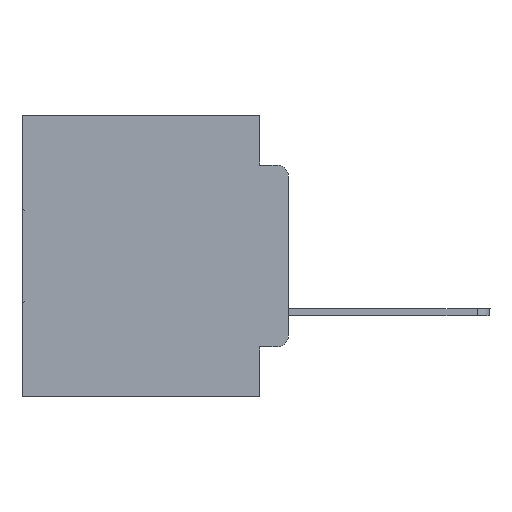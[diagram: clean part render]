
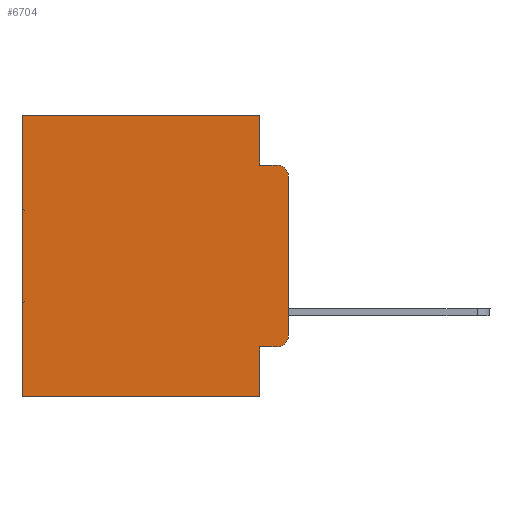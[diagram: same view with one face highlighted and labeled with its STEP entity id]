
A CAD part, left-side view. The second image highlights one B-rep face of the part: STEP entity #6704.
In plain terms, the highlighted planar face has unit normal (-1, 0, 0).
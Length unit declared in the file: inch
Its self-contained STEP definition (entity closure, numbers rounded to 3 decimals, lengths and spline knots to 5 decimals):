
#90 = AXIS2_PLACEMENT_3D ( 'NONE', #8830, #5706, #25961 ) ;
#226 = DIRECTION ( 'NONE',  ( 0., 0., -1. ) ) ;
#318 = DIRECTION ( 'NONE',  ( 0., -1., 0. ) ) ;
#377 = ORIENTED_EDGE ( 'NONE', *, *, #26750, .F. ) ;
#945 = EDGE_CURVE ( 'NONE', #11277, #2841, #8264, .T. ) ;
#1749 = VECTOR ( 'NONE', #15007, 39.37008 ) ;
#2358 = VERTEX_POINT ( 'NONE', #23683 ) ;
#2548 = DIRECTION ( 'NONE',  ( -1., 0., 0. ) ) ;
#2841 = VERTEX_POINT ( 'NONE', #30190 ) ;
#4095 = VERTEX_POINT ( 'NONE', #14268 ) ;
#5706 = DIRECTION ( 'NONE',  ( 1., 0., 0. ) ) ;
#6704 = ADVANCED_FACE ( 'NONE', ( #26264 ), #23604, .F. ) ;
#6793 = ORIENTED_EDGE ( 'NONE', *, *, #945, .T. ) ;
#7123 = CIRCLE ( 'NONE', #26198, 0.02 ) ;
#7541 = DIRECTION ( 'NONE',  ( 0., 0., -1. ) ) ;
#7926 = VERTEX_POINT ( 'NONE', #11669 ) ;
#8264 = CIRCLE ( 'NONE', #11967, 0.02 ) ;
#8830 = CARTESIAN_POINT ( 'NONE',  ( 0.298, 0., 0. ) ) ;
#8970 = CARTESIAN_POINT ( 'NONE',  ( 0.298, 0.051, -0.5 ) ) ;
#9773 = VERTEX_POINT ( 'NONE', #14271 ) ;
#9861 = CARTESIAN_POINT ( 'NONE',  ( 0.298, 0.473, 0. ) ) ;
#10198 = EDGE_CURVE ( 'NONE', #11277, #2358, #32067, .T. ) ;
#10336 = CARTESIAN_POINT ( 'NONE',  ( 0.298, 0., 0. ) ) ;
#11277 = VERTEX_POINT ( 'NONE', #15738 ) ;
#11669 = CARTESIAN_POINT ( 'NONE',  ( 0.298, 0.051, -0.0885 ) ) ;
#11847 = EDGE_CURVE ( 'NONE', #4095, #7926, #25296, .T. ) ;
#11967 = AXIS2_PLACEMENT_3D ( 'NONE', #25267, #2548, #226 ) ;
#12024 = CARTESIAN_POINT ( 'NONE',  ( 0.298, 0., -0.5 ) ) ;
#12555 = VECTOR ( 'NONE', #22313, 39.37008 ) ;
#12755 = ORIENTED_EDGE ( 'NONE', *, *, #15645, .T. ) ;
#12831 = DIRECTION ( 'NONE',  ( 0., 0., -1. ) ) ;
#12907 = LINE ( 'NONE', #23021, #32037 ) ;
#13160 = EDGE_CURVE ( 'NONE', #21122, #24036, #25468, .T. ) ;
#13433 = DIRECTION ( 'NONE',  ( 0., -1., 0. ) ) ;
#13849 = EDGE_LOOP ( 'NONE', ( #21190, #6793, #19147, #27685, #12755, #30807, #377, #22683, #17569, #29836 ) ) ;
#14147 = CARTESIAN_POINT ( 'NONE',  ( 0.298, 0.473, -0.5 ) ) ;
#14268 = CARTESIAN_POINT ( 'NONE',  ( 0.298, 0.051, 0. ) ) ;
#14271 = CARTESIAN_POINT ( 'NONE',  ( 0.298, 0.051, -0.4115 ) ) ;
#15005 = DIRECTION ( 'NONE',  ( 0., 1., 0. ) ) ;
#15007 = DIRECTION ( 'NONE',  ( 0., 0., -1. ) ) ;
#15645 = EDGE_CURVE ( 'NONE', #4095, #21122, #18136, .T. ) ;
#15738 = CARTESIAN_POINT ( 'NONE',  ( 0.298, 0., -0.1085 ) ) ;
#16274 = VECTOR ( 'NONE', #15005, 39.37008 ) ;
#17162 = VERTEX_POINT ( 'NONE', #24941 ) ;
#17569 = ORIENTED_EDGE ( 'NONE', *, *, #23483, .T. ) ;
#18136 = LINE ( 'NONE', #30232, #16274 ) ;
#19147 = ORIENTED_EDGE ( 'NONE', *, *, #20610, .F. ) ;
#19467 = CARTESIAN_POINT ( 'NONE',  ( 0.298, 0.473, 0. ) ) ;
#20610 = EDGE_CURVE ( 'NONE', #7926, #2841, #26049, .T. ) ;
#21122 = VERTEX_POINT ( 'NONE', #19467 ) ;
#21190 = ORIENTED_EDGE ( 'NONE', *, *, #10198, .F. ) ;
#22014 = VECTOR ( 'NONE', #12831, 39.37008 ) ;
#22313 = DIRECTION ( 'NONE',  ( 0., 1., 0. ) ) ;
#22454 = EDGE_CURVE ( 'NONE', #17162, #2358, #7123, .T. ) ;
#22683 = ORIENTED_EDGE ( 'NONE', *, *, #23803, .F. ) ;
#22791 = CARTESIAN_POINT ( 'NONE',  ( 0.298, 0.051, 0. ) ) ;
#23021 = CARTESIAN_POINT ( 'NONE',  ( 0.298, 0.051, -0.4115 ) ) ;
#23483 = EDGE_CURVE ( 'NONE', #9773, #17162, #12907, .T. ) ;
#23519 = DIRECTION ( 'NONE',  ( 0., 0., -1. ) ) ;
#23604 = PLANE ( 'NONE',  #90 ) ;
#23683 = CARTESIAN_POINT ( 'NONE',  ( 0.298, 0., -0.3915 ) ) ;
#23803 = EDGE_CURVE ( 'NONE', #9773, #29798, #30231, .T. ) ;
#23871 = CARTESIAN_POINT ( 'NONE',  ( 0.298, 0.051, -0.0885 ) ) ;
#24036 = VERTEX_POINT ( 'NONE', #14147 ) ;
#24639 = VECTOR ( 'NONE', #27903, 39.37008 ) ;
#24882 = VECTOR ( 'NONE', #13433, 39.37008 ) ;
#24941 = CARTESIAN_POINT ( 'NONE',  ( 0.298, 0.02, -0.4115 ) ) ;
#25267 = CARTESIAN_POINT ( 'NONE',  ( 0.298, 0.02, -0.1085 ) ) ;
#25296 = LINE ( 'NONE', #22791, #1749 ) ;
#25457 = CARTESIAN_POINT ( 'NONE',  ( 0.298, 0.051, 0. ) ) ;
#25468 = LINE ( 'NONE', #9861, #25872 ) ;
#25872 = VECTOR ( 'NONE', #7541, 39.37008 ) ;
#25961 = DIRECTION ( 'NONE',  ( 0., 0., -1. ) ) ;
#26049 = LINE ( 'NONE', #23871, #24882 ) ;
#26198 = AXIS2_PLACEMENT_3D ( 'NONE', #30637, #30959, #23519 ) ;
#26264 = FACE_OUTER_BOUND ( 'NONE', #13849, .T. ) ;
#26750 = EDGE_CURVE ( 'NONE', #29798, #24036, #27129, .T. ) ;
#27129 = LINE ( 'NONE', #12024, #12555 ) ;
#27685 = ORIENTED_EDGE ( 'NONE', *, *, #11847, .F. ) ;
#27903 = DIRECTION ( 'NONE',  ( 0., 0., -1. ) ) ;
#29798 = VERTEX_POINT ( 'NONE', #8970 ) ;
#29836 = ORIENTED_EDGE ( 'NONE', *, *, #22454, .T. ) ;
#30190 = CARTESIAN_POINT ( 'NONE',  ( 0.298, 0.02, -0.0885 ) ) ;
#30231 = LINE ( 'NONE', #25457, #22014 ) ;
#30232 = CARTESIAN_POINT ( 'NONE',  ( 0.298, 0., 0. ) ) ;
#30637 = CARTESIAN_POINT ( 'NONE',  ( 0.298, 0.02, -0.3915 ) ) ;
#30807 = ORIENTED_EDGE ( 'NONE', *, *, #13160, .T. ) ;
#30959 = DIRECTION ( 'NONE',  ( -1., 0., 0. ) ) ;
#32037 = VECTOR ( 'NONE', #318, 39.37008 ) ;
#32067 = LINE ( 'NONE', #10336, #24639 ) ;
